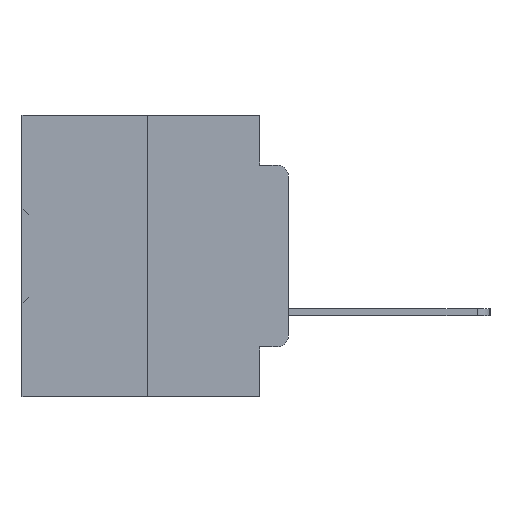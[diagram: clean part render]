
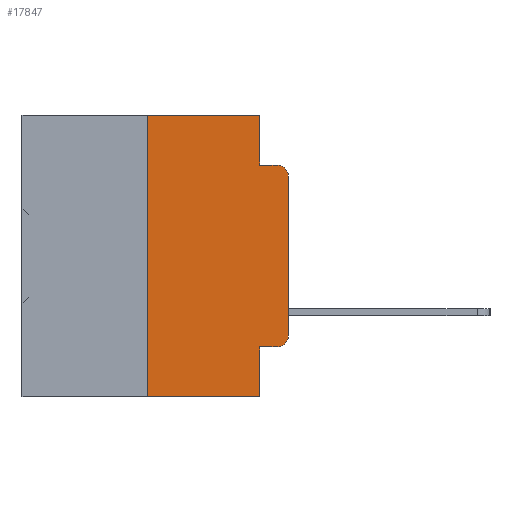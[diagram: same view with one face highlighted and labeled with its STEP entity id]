
A CAD part, left-side view. The second image highlights one B-rep face of the part: STEP entity #17847.
In plain terms, the highlighted planar face has unit normal (-1, 0, 0).
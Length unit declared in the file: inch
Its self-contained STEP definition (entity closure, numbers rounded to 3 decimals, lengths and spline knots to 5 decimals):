
#458 = LINE ( 'NONE', #20201, #32023 ) ;
#611 = VECTOR ( 'NONE', #37800, 39.37008 ) ;
#1062 = DIRECTION ( 'NONE',  ( 0., -1., 0. ) ) ;
#2488 = EDGE_CURVE ( 'NONE', #5174, #37593, #458, .T. ) ;
#3064 = DIRECTION ( 'NONE',  ( 0., 0., -1. ) ) ;
#3160 = LINE ( 'NONE', #25638, #18118 ) ;
#3393 = VERTEX_POINT ( 'NONE', #7676 ) ;
#3582 = ORIENTED_EDGE ( 'NONE', *, *, #9928, .T. ) ;
#3660 = CARTESIAN_POINT ( 'NONE',  ( 0., 0.02, -0.4115 ) ) ;
#3672 = CARTESIAN_POINT ( 'NONE',  ( 0., 0.25, -0.5 ) ) ;
#3705 = VERTEX_POINT ( 'NONE', #7939 ) ;
#3826 = DIRECTION ( 'NONE',  ( 0., -1., 0. ) ) ;
#3910 = CIRCLE ( 'NONE', #23823, 0.02 ) ;
#5006 = ORIENTED_EDGE ( 'NONE', *, *, #36656, .F. ) ;
#5174 = VERTEX_POINT ( 'NONE', #3672 ) ;
#5589 = VECTOR ( 'NONE', #16600, 39.37008 ) ;
#5909 = DIRECTION ( 'NONE',  ( 0., 0., -1. ) ) ;
#6059 = CARTESIAN_POINT ( 'NONE',  ( 0., 0.051, -0.4115 ) ) ;
#7326 = CARTESIAN_POINT ( 'NONE',  ( 0., 0.051, -0.5 ) ) ;
#7676 = CARTESIAN_POINT ( 'NONE',  ( 0., 0.051, 0. ) ) ;
#7684 = CARTESIAN_POINT ( 'NONE',  ( 0., 0.02, -0.3915 ) ) ;
#7939 = CARTESIAN_POINT ( 'NONE',  ( 0., 0.02, -0.0885 ) ) ;
#8141 = DIRECTION ( 'NONE',  ( 1., 0., 0. ) ) ;
#8916 = LINE ( 'NONE', #9935, #31518 ) ;
#9078 = EDGE_LOOP ( 'NONE', ( #19009, #30004, #9271, #35553, #5006, #16700, #3582, #14439, #22190, #20835 ) ) ;
#9271 = ORIENTED_EDGE ( 'NONE', *, *, #12593, .F. ) ;
#9532 = CARTESIAN_POINT ( 'NONE',  ( 0., 0., -0.1085 ) ) ;
#9928 = EDGE_CURVE ( 'NONE', #5174, #29328, #24315, .T. ) ;
#9935 = CARTESIAN_POINT ( 'NONE',  ( 0., 0.473, 0. ) ) ;
#10625 = EDGE_CURVE ( 'NONE', #3393, #14728, #22886, .T. ) ;
#10727 = DIRECTION ( 'NONE',  ( 0., 0., -1. ) ) ;
#11149 = DIRECTION ( 'NONE',  ( 0., -1., 0. ) ) ;
#12198 = FACE_OUTER_BOUND ( 'NONE', #9078, .T. ) ;
#12537 = LINE ( 'NONE', #27408, #28141 ) ;
#12549 = AXIS2_PLACEMENT_3D ( 'NONE', #7684, #28305, #10727 ) ;
#12593 = EDGE_CURVE ( 'NONE', #14728, #3705, #12537, .T. ) ;
#12624 = LINE ( 'NONE', #20687, #34265 ) ;
#13044 = VERTEX_POINT ( 'NONE', #6059 ) ;
#14272 = CARTESIAN_POINT ( 'NONE',  ( 0., 0.473, -0.5 ) ) ;
#14439 = ORIENTED_EDGE ( 'NONE', *, *, #36988, .F. ) ;
#14728 = VERTEX_POINT ( 'NONE', #29244 ) ;
#15024 = VERTEX_POINT ( 'NONE', #3660 ) ;
#15759 = CARTESIAN_POINT ( 'NONE',  ( 0., 0.02, -0.1085 ) ) ;
#16600 = DIRECTION ( 'NONE',  ( 0., 0., 1. ) ) ;
#16700 = ORIENTED_EDGE ( 'NONE', *, *, #2488, .F. ) ;
#17847 = ADVANCED_FACE ( 'NONE', ( #12198 ), #19903, .F. ) ;
#18118 = VECTOR ( 'NONE', #11149, 39.37008 ) ;
#18225 = CARTESIAN_POINT ( 'NONE',  ( 0., 0.25, 0. ) ) ;
#18700 = DIRECTION ( 'NONE',  ( 0., 0., -1. ) ) ;
#19009 = ORIENTED_EDGE ( 'NONE', *, *, #26333, .T. ) ;
#19903 = PLANE ( 'NONE',  #33163 ) ;
#20201 = CARTESIAN_POINT ( 'NONE',  ( 0., 0.25, 0. ) ) ;
#20434 = EDGE_CURVE ( 'NONE', #34145, #3705, #3910, .T. ) ;
#20687 = CARTESIAN_POINT ( 'NONE',  ( 0., 0.051, 0. ) ) ;
#20751 = CARTESIAN_POINT ( 'NONE',  ( 0., 0.051, 0. ) ) ;
#20835 = ORIENTED_EDGE ( 'NONE', *, *, #21169, .T. ) ;
#21169 = EDGE_CURVE ( 'NONE', #15024, #22717, #24816, .T. ) ;
#21361 = LINE ( 'NONE', #37199, #5589 ) ;
#21943 = VECTOR ( 'NONE', #3064, 39.37008 ) ;
#22190 = ORIENTED_EDGE ( 'NONE', *, *, #27060, .T. ) ;
#22717 = VERTEX_POINT ( 'NONE', #37781 ) ;
#22886 = LINE ( 'NONE', #20751, #21943 ) ;
#23823 = AXIS2_PLACEMENT_3D ( 'NONE', #15759, #36343, #18700 ) ;
#24315 = LINE ( 'NONE', #14272, #611 ) ;
#24816 = CIRCLE ( 'NONE', #12549, 0.02 ) ;
#25638 = CARTESIAN_POINT ( 'NONE',  ( 0., 0.051, -0.4115 ) ) ;
#25778 = CARTESIAN_POINT ( 'NONE',  ( 0., 0.473, 0. ) ) ;
#26333 = EDGE_CURVE ( 'NONE', #22717, #34145, #21361, .T. ) ;
#27060 = EDGE_CURVE ( 'NONE', #13044, #15024, #3160, .T. ) ;
#27408 = CARTESIAN_POINT ( 'NONE',  ( 0., 0.051, -0.0885 ) ) ;
#28141 = VECTOR ( 'NONE', #3826, 39.37008 ) ;
#28305 = DIRECTION ( 'NONE',  ( -1., 0., 0. ) ) ;
#28769 = DIRECTION ( 'NONE',  ( 0., 0., -1. ) ) ;
#29244 = CARTESIAN_POINT ( 'NONE',  ( 0., 0.051, -0.0885 ) ) ;
#29328 = VERTEX_POINT ( 'NONE', #7326 ) ;
#30004 = ORIENTED_EDGE ( 'NONE', *, *, #20434, .T. ) ;
#30470 = DIRECTION ( 'NONE',  ( 0., 0., 1. ) ) ;
#31518 = VECTOR ( 'NONE', #1062, 39.37008 ) ;
#32023 = VECTOR ( 'NONE', #30470, 39.37008 ) ;
#33163 = AXIS2_PLACEMENT_3D ( 'NONE', #25778, #8141, #28769 ) ;
#34145 = VERTEX_POINT ( 'NONE', #9532 ) ;
#34265 = VECTOR ( 'NONE', #5909, 39.37008 ) ;
#35553 = ORIENTED_EDGE ( 'NONE', *, *, #10625, .F. ) ;
#36343 = DIRECTION ( 'NONE',  ( -1., 0., 0. ) ) ;
#36656 = EDGE_CURVE ( 'NONE', #37593, #3393, #8916, .T. ) ;
#36988 = EDGE_CURVE ( 'NONE', #13044, #29328, #12624, .T. ) ;
#37199 = CARTESIAN_POINT ( 'NONE',  ( 0., 0., 0. ) ) ;
#37593 = VERTEX_POINT ( 'NONE', #18225 ) ;
#37781 = CARTESIAN_POINT ( 'NONE',  ( 0., 0., -0.3915 ) ) ;
#37800 = DIRECTION ( 'NONE',  ( 0., -1., 0. ) ) ;
